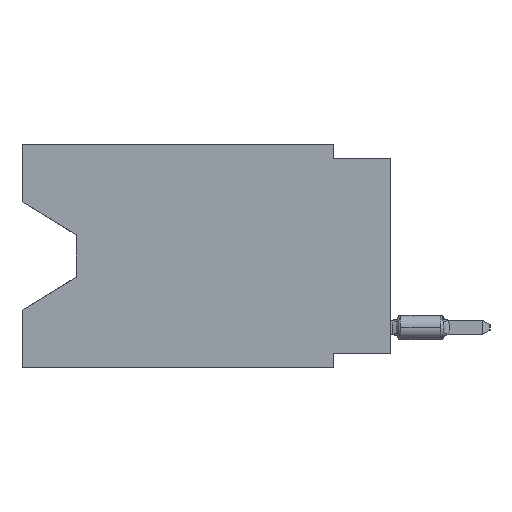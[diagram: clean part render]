
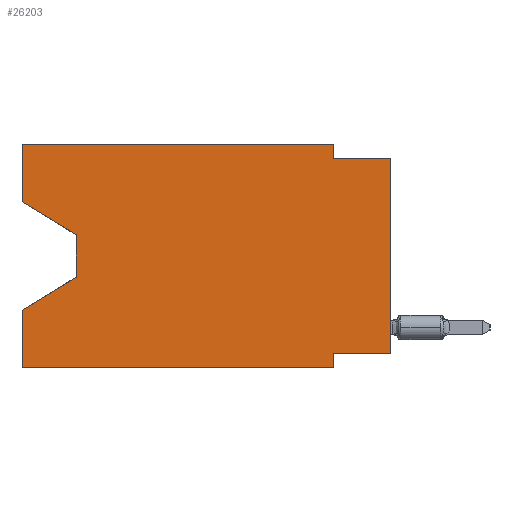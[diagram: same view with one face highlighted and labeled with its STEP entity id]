
A CAD part, left-side view. The second image highlights one B-rep face of the part: STEP entity #26203.
In plain terms, the highlighted planar face has unit normal (-1, 0, 0).
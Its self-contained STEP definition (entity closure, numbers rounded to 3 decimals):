
#349 = LINE ( 'NONE', #10222, #26060 ) ;
#575 = VERTEX_POINT ( 'NONE', #23982 ) ;
#690 = VERTEX_POINT ( 'NONE', #2755 ) ;
#1292 = ORIENTED_EDGE ( 'NONE', *, *, #7936, .F. ) ;
#2755 = CARTESIAN_POINT ( 'NONE',  ( 0., 0., -9.271 ) ) ;
#3450 = VERTEX_POINT ( 'NONE', #21715 ) ;
#3486 = DIRECTION ( 'NONE',  ( 0., 0., -1. ) ) ;
#3487 = CARTESIAN_POINT ( 'NONE',  ( 0., 13.97, -4.013 ) ) ;
#3593 = LINE ( 'NONE', #5886, #13038 ) ;
#4188 = LINE ( 'NONE', #8891, #19254 ) ;
#4196 = CARTESIAN_POINT ( 'NONE',  ( 0., 16.383, 0. ) ) ;
#4264 = DIRECTION ( 'NONE',  ( 0., 0., 1. ) ) ;
#4706 = CARTESIAN_POINT ( 'NONE',  ( 0., 0., -9.271 ) ) ;
#4977 = VERTEX_POINT ( 'NONE', #15507 ) ;
#5202 = CARTESIAN_POINT ( 'NONE',  ( 0., 2.54, -9.906 ) ) ;
#5348 = ORIENTED_EDGE ( 'NONE', *, *, #25888, .F. ) ;
#5460 = VERTEX_POINT ( 'NONE', #25365 ) ;
#5631 = VECTOR ( 'NONE', #30510, 1000. ) ;
#5886 = CARTESIAN_POINT ( 'NONE',  ( 0., 2.54, -9.906 ) ) ;
#5962 = VECTOR ( 'NONE', #19507, 1000. ) ;
#6299 = VECTOR ( 'NONE', #12065, 1000. ) ;
#6380 = CARTESIAN_POINT ( 'NONE',  ( 0., 0., 0. ) ) ;
#6655 = VERTEX_POINT ( 'NONE', #4196 ) ;
#6994 = CARTESIAN_POINT ( 'NONE',  ( 0., 16.383, -7.36 ) ) ;
#7572 = VERTEX_POINT ( 'NONE', #29069 ) ;
#7936 = EDGE_CURVE ( 'NONE', #690, #5460, #14102, .T. ) ;
#8395 = VECTOR ( 'NONE', #4264, 1000. ) ;
#8884 = VECTOR ( 'NONE', #31449, 1000. ) ;
#8891 = CARTESIAN_POINT ( 'NONE',  ( 0., 16.383, -2.546 ) ) ;
#9198 = EDGE_CURVE ( 'NONE', #31447, #7572, #28396, .T. ) ;
#9995 = ORIENTED_EDGE ( 'NONE', *, *, #26598, .F. ) ;
#10222 = CARTESIAN_POINT ( 'NONE',  ( 0., 13.97, -5.893 ) ) ;
#10267 = ORIENTED_EDGE ( 'NONE', *, *, #29227, .T. ) ;
#10994 = EDGE_CURVE ( 'NONE', #6655, #29781, #24558, .T. ) ;
#11836 = VERTEX_POINT ( 'NONE', #6994 ) ;
#12004 = DIRECTION ( 'NONE',  ( 0., 0., 1. ) ) ;
#12065 = DIRECTION ( 'NONE',  ( 0., 0., 1. ) ) ;
#12925 = CARTESIAN_POINT ( 'NONE',  ( 0., 2.54, 0. ) ) ;
#12991 = VERTEX_POINT ( 'NONE', #25730 ) ;
#13038 = VECTOR ( 'NONE', #15745, 1000. ) ;
#13193 = ORIENTED_EDGE ( 'NONE', *, *, #28079, .F. ) ;
#13849 = CARTESIAN_POINT ( 'NONE',  ( 0., 16.383, -9.906 ) ) ;
#14102 = LINE ( 'NONE', #4706, #29410 ) ;
#14305 = ORIENTED_EDGE ( 'NONE', *, *, #28216, .T. ) ;
#14586 = AXIS2_PLACEMENT_3D ( 'NONE', #18218, #25668, #3486 ) ;
#15133 = VECTOR ( 'NONE', #19919, 1000. ) ;
#15154 = EDGE_CURVE ( 'NONE', #690, #12991, #19323, .T. ) ;
#15507 = CARTESIAN_POINT ( 'NONE',  ( 0., 16.383, -2.546 ) ) ;
#15569 = EDGE_CURVE ( 'NONE', #3450, #12991, #19109, .T. ) ;
#15745 = DIRECTION ( 'NONE',  ( 0., 0., -1. ) ) ;
#15787 = FACE_OUTER_BOUND ( 'NONE', #22670, .T. ) ;
#16434 = LINE ( 'NONE', #13849, #5962 ) ;
#16601 = CARTESIAN_POINT ( 'NONE',  ( 0., 16.383, 0. ) ) ;
#16810 = ORIENTED_EDGE ( 'NONE', *, *, #9198, .T. ) ;
#18172 = VERTEX_POINT ( 'NONE', #5202 ) ;
#18218 = CARTESIAN_POINT ( 'NONE',  ( 0., 16.383, 0. ) ) ;
#18605 = DIRECTION ( 'NONE',  ( 0., -0.855, -0.519 ) ) ;
#18718 = CARTESIAN_POINT ( 'NONE',  ( 0., 13.97, -4.013 ) ) ;
#18846 = CARTESIAN_POINT ( 'NONE',  ( 0., 2.54, 0. ) ) ;
#19109 = LINE ( 'NONE', #22015, #15133 ) ;
#19254 = VECTOR ( 'NONE', #18605, 1000. ) ;
#19323 = LINE ( 'NONE', #6380, #8395 ) ;
#19366 = LINE ( 'NONE', #16601, #6299 ) ;
#19507 = DIRECTION ( 'NONE',  ( 0., -1., 0. ) ) ;
#19919 = DIRECTION ( 'NONE',  ( 0., -1., 0. ) ) ;
#20763 = ORIENTED_EDGE ( 'NONE', *, *, #26218, .F. ) ;
#21715 = CARTESIAN_POINT ( 'NONE',  ( 0., 2.54, -0.635 ) ) ;
#22015 = CARTESIAN_POINT ( 'NONE',  ( 0., 0., -0.635 ) ) ;
#22420 = VECTOR ( 'NONE', #12004, 1000. ) ;
#22670 = EDGE_LOOP ( 'NONE', ( #30659, #16810, #14305, #13193, #10267, #9995, #1292, #25197, #27571, #20763, #23469, #5348 ) ) ;
#23469 = ORIENTED_EDGE ( 'NONE', *, *, #10994, .F. ) ;
#23982 = CARTESIAN_POINT ( 'NONE',  ( 0., 16.383, -9.906 ) ) ;
#24481 = DIRECTION ( 'NONE',  ( 0., 1., 0. ) ) ;
#24558 = LINE ( 'NONE', #24863, #25865 ) ;
#24863 = CARTESIAN_POINT ( 'NONE',  ( 0., 16.383, 0. ) ) ;
#25197 = ORIENTED_EDGE ( 'NONE', *, *, #15154, .T. ) ;
#25365 = CARTESIAN_POINT ( 'NONE',  ( 0., 2.54, -9.271 ) ) ;
#25668 = DIRECTION ( 'NONE',  ( 1., 0., 0. ) ) ;
#25730 = CARTESIAN_POINT ( 'NONE',  ( 0., 0., -0.635 ) ) ;
#25865 = VECTOR ( 'NONE', #31651, 1000. ) ;
#25888 = EDGE_CURVE ( 'NONE', #4977, #6655, #19366, .T. ) ;
#26060 = VECTOR ( 'NONE', #29954, 1000. ) ;
#26203 = ADVANCED_FACE ( 'NONE', ( #15787 ), #30508, .F. ) ;
#26218 = EDGE_CURVE ( 'NONE', #29781, #3450, #26612, .T. ) ;
#26598 = EDGE_CURVE ( 'NONE', #5460, #18172, #3593, .T. ) ;
#26612 = LINE ( 'NONE', #18846, #8884 ) ;
#27034 = EDGE_CURVE ( 'NONE', #4977, #31447, #4188, .T. ) ;
#27214 = CARTESIAN_POINT ( 'NONE',  ( 0., 16.383, 0. ) ) ;
#27571 = ORIENTED_EDGE ( 'NONE', *, *, #15569, .F. ) ;
#28079 = EDGE_CURVE ( 'NONE', #575, #11836, #29642, .T. ) ;
#28216 = EDGE_CURVE ( 'NONE', #7572, #11836, #349, .T. ) ;
#28396 = LINE ( 'NONE', #3487, #5631 ) ;
#29069 = CARTESIAN_POINT ( 'NONE',  ( 0., 13.97, -5.893 ) ) ;
#29227 = EDGE_CURVE ( 'NONE', #575, #18172, #16434, .T. ) ;
#29410 = VECTOR ( 'NONE', #24481, 1000. ) ;
#29642 = LINE ( 'NONE', #27214, #22420 ) ;
#29781 = VERTEX_POINT ( 'NONE', #12925 ) ;
#29954 = DIRECTION ( 'NONE',  ( 0., 0.855, -0.519 ) ) ;
#30508 = PLANE ( 'NONE',  #14586 ) ;
#30510 = DIRECTION ( 'NONE',  ( 0., 0., -1. ) ) ;
#30659 = ORIENTED_EDGE ( 'NONE', *, *, #27034, .T. ) ;
#31447 = VERTEX_POINT ( 'NONE', #18718 ) ;
#31449 = DIRECTION ( 'NONE',  ( 0., 0., -1. ) ) ;
#31651 = DIRECTION ( 'NONE',  ( 0., -1., 0. ) ) ;
